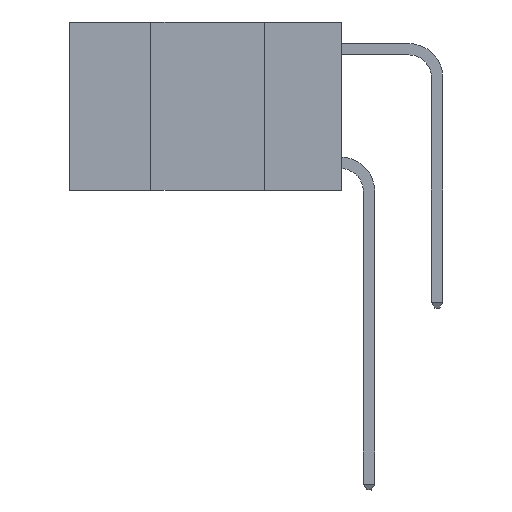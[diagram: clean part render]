
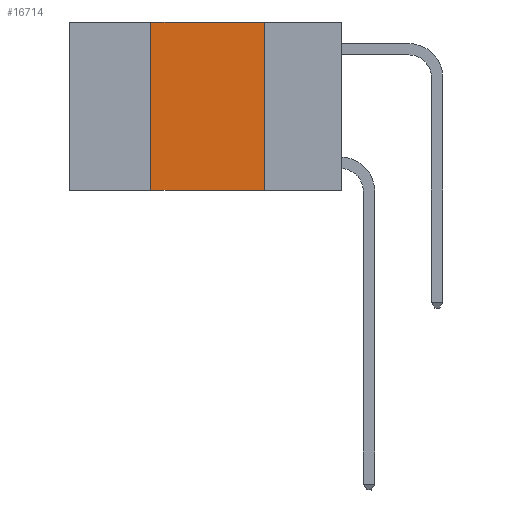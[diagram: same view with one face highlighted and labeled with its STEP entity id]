
A CAD part, left-side view. The second image highlights one B-rep face of the part: STEP entity #16714.
In plain terms, the highlighted planar face has unit normal (-1, 0, 0).
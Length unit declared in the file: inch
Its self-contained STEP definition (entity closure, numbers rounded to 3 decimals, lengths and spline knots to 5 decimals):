
#1000 = EDGE_CURVE ( 'NONE', #5963, #21087, #2372, .T. ) ;
#1341 = DIRECTION ( 'NONE',  ( 0., 0., -1. ) ) ;
#1451 = VECTOR ( 'NONE', #18142, 39.37008 ) ;
#2042 = EDGE_CURVE ( 'NONE', #20405, #5326, #10323, .T. ) ;
#2102 = CARTESIAN_POINT ( 'NONE',  ( 0., 0.17, -0.37 ) ) ;
#2372 = LINE ( 'NONE', #5136, #17372 ) ;
#2778 = ORIENTED_EDGE ( 'NONE', *, *, #1000, .F. ) ;
#3271 = DIRECTION ( 'NONE',  ( 0., -1., 0. ) ) ;
#3455 = ORIENTED_EDGE ( 'NONE', *, *, #8828, .F. ) ;
#3634 = FACE_OUTER_BOUND ( 'NONE', #7969, .T. ) ;
#4453 = VECTOR ( 'NONE', #19521, 39.37008 ) ;
#5136 = CARTESIAN_POINT ( 'NONE',  ( 0., 0.6, 0. ) ) ;
#5326 = VERTEX_POINT ( 'NONE', #2102 ) ;
#5963 = VERTEX_POINT ( 'NONE', #13999 ) ;
#6225 = ORIENTED_EDGE ( 'NONE', *, *, #2042, .T. ) ;
#7969 = EDGE_LOOP ( 'NONE', ( #24979, #2778, #3455, #6225 ) ) ;
#8775 = DIRECTION ( 'NONE',  ( 0., 0., 1. ) ) ;
#8828 = EDGE_CURVE ( 'NONE', #20405, #5963, #12800, .T. ) ;
#9080 = PLANE ( 'NONE',  #20757 ) ;
#10323 = LINE ( 'NONE', #19843, #4453 ) ;
#12800 = LINE ( 'NONE', #20379, #19168 ) ;
#13069 = DIRECTION ( 'NONE',  ( 1., 0., 0. ) ) ;
#13999 = CARTESIAN_POINT ( 'NONE',  ( 0., 0.42, 0. ) ) ;
#15337 = CARTESIAN_POINT ( 'NONE',  ( 0., 0.42, -0.37 ) ) ;
#16714 = ADVANCED_FACE ( 'NONE', ( #3634 ), #9080, .F. ) ;
#17372 = VECTOR ( 'NONE', #3271, 39.37008 ) ;
#17637 = LINE ( 'NONE', #23985, #1451 ) ;
#18142 = DIRECTION ( 'NONE',  ( 0., 0., -1. ) ) ;
#19168 = VECTOR ( 'NONE', #8775, 39.37008 ) ;
#19521 = DIRECTION ( 'NONE',  ( 0., -1., 0. ) ) ;
#19843 = CARTESIAN_POINT ( 'NONE',  ( 0., 0.6, -0.37 ) ) ;
#20379 = CARTESIAN_POINT ( 'NONE',  ( 0., 0.42, 0. ) ) ;
#20405 = VERTEX_POINT ( 'NONE', #15337 ) ;
#20757 = AXIS2_PLACEMENT_3D ( 'NONE', #24667, #13069, #1341 ) ;
#21087 = VERTEX_POINT ( 'NONE', #25103 ) ;
#23985 = CARTESIAN_POINT ( 'NONE',  ( 0., 0.17, 0. ) ) ;
#24667 = CARTESIAN_POINT ( 'NONE',  ( 0., 0.6, 0. ) ) ;
#24979 = ORIENTED_EDGE ( 'NONE', *, *, #25009, .F. ) ;
#25009 = EDGE_CURVE ( 'NONE', #21087, #5326, #17637, .T. ) ;
#25103 = CARTESIAN_POINT ( 'NONE',  ( 0., 0.17, 0. ) ) ;
